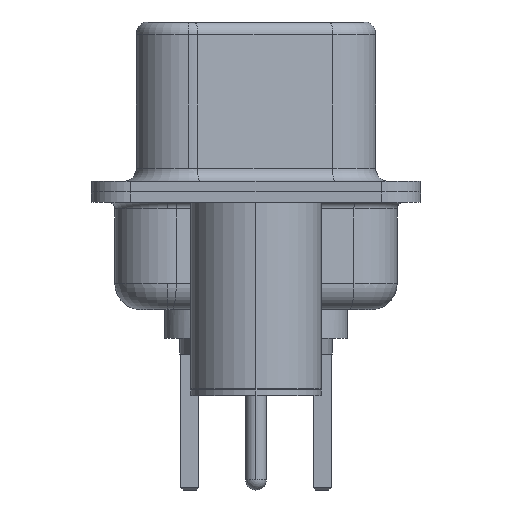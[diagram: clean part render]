
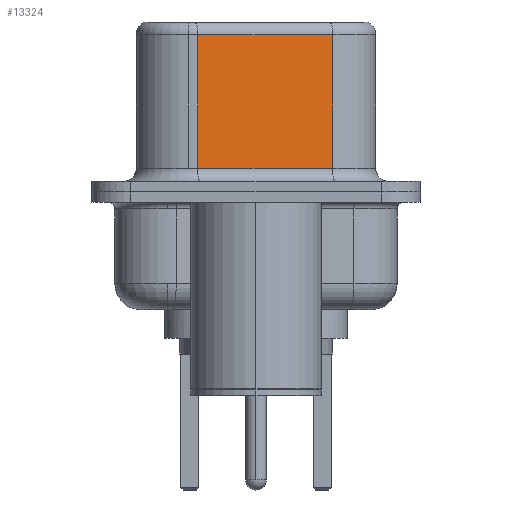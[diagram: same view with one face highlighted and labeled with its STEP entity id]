
A CAD part, left-side view. The second image highlights one B-rep face of the part: STEP entity #13324.
In plain terms, the highlighted planar face has unit normal (-0.985, -0.174, 0).
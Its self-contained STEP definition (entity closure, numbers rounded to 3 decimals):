
#1117 = LINE ( 'NONE', #4786, #13855 ) ;
#1352 = ORIENTED_EDGE ( 'NONE', *, *, #9523, .F. ) ;
#1458 = VERTEX_POINT ( 'NONE', #7722 ) ;
#1542 = EDGE_CURVE ( 'NONE', #19446, #5859, #8923, .T. ) ;
#2715 = DIRECTION ( 'NONE',  ( 0., 0., -1. ) ) ;
#2764 = LINE ( 'NONE', #14243, #15301 ) ;
#3980 = EDGE_LOOP ( 'NONE', ( #1352, #11984, #18361, #4010 ) ) ;
#4010 = ORIENTED_EDGE ( 'NONE', *, *, #9628, .T. ) ;
#4279 = VECTOR ( 'NONE', #18495, 1000. ) ;
#4786 = CARTESIAN_POINT ( 'NONE',  ( 4.585, -2.927, 0.9 ) ) ;
#5501 = PLANE ( 'NONE',  #6978 ) ;
#5643 = CARTESIAN_POINT ( 'NONE',  ( 4.585, -2.927, 6.52 ) ) ;
#5859 = VERTEX_POINT ( 'NONE', #12053 ) ;
#6505 = DIRECTION ( 'NONE',  ( 0.174, -0.985, 0. ) ) ;
#6978 = AXIS2_PLACEMENT_3D ( 'NONE', #5643, #7347, #18565 ) ;
#7347 = DIRECTION ( 'NONE',  ( 0.985, 0.174, 0. ) ) ;
#7722 = CARTESIAN_POINT ( 'NONE',  ( 4.585, -2.927, 0.9 ) ) ;
#7804 = VERTEX_POINT ( 'NONE', #19447 ) ;
#8410 = VECTOR ( 'NONE', #12442, 1000. ) ;
#8730 = LINE ( 'NONE', #8925, #4279 ) ;
#8923 = LINE ( 'NONE', #10769, #8410 ) ;
#8925 = CARTESIAN_POINT ( 'NONE',  ( 4.585, -2.927, 6.02 ) ) ;
#9523 = EDGE_CURVE ( 'NONE', #7804, #1458, #2764, .T. ) ;
#9628 = EDGE_CURVE ( 'NONE', #5859, #1458, #1117, .T. ) ;
#10769 = CARTESIAN_POINT ( 'NONE',  ( 3.675, 2.233, 6.52 ) ) ;
#11984 = ORIENTED_EDGE ( 'NONE', *, *, #17636, .T. ) ;
#12053 = CARTESIAN_POINT ( 'NONE',  ( 3.675, 2.233, 0.9 ) ) ;
#12105 = CARTESIAN_POINT ( 'NONE',  ( 3.675, 2.233, 6.02 ) ) ;
#12442 = DIRECTION ( 'NONE',  ( 0., 0., -1. ) ) ;
#13324 = ADVANCED_FACE ( 'NONE', ( #17156 ), #5501, .F. ) ;
#13855 = VECTOR ( 'NONE', #6505, 1000. ) ;
#14243 = CARTESIAN_POINT ( 'NONE',  ( 4.585, -2.927, 6.52 ) ) ;
#15301 = VECTOR ( 'NONE', #2715, 1000. ) ;
#17156 = FACE_OUTER_BOUND ( 'NONE', #3980, .T. ) ;
#17636 = EDGE_CURVE ( 'NONE', #7804, #19446, #8730, .T. ) ;
#18361 = ORIENTED_EDGE ( 'NONE', *, *, #1542, .T. ) ;
#18495 = DIRECTION ( 'NONE',  ( -0.174, 0.985, 0. ) ) ;
#18565 = DIRECTION ( 'NONE',  ( -0.174, 0.985, 0. ) ) ;
#19446 = VERTEX_POINT ( 'NONE', #12105 ) ;
#19447 = CARTESIAN_POINT ( 'NONE',  ( 4.585, -2.927, 6.02 ) ) ;
